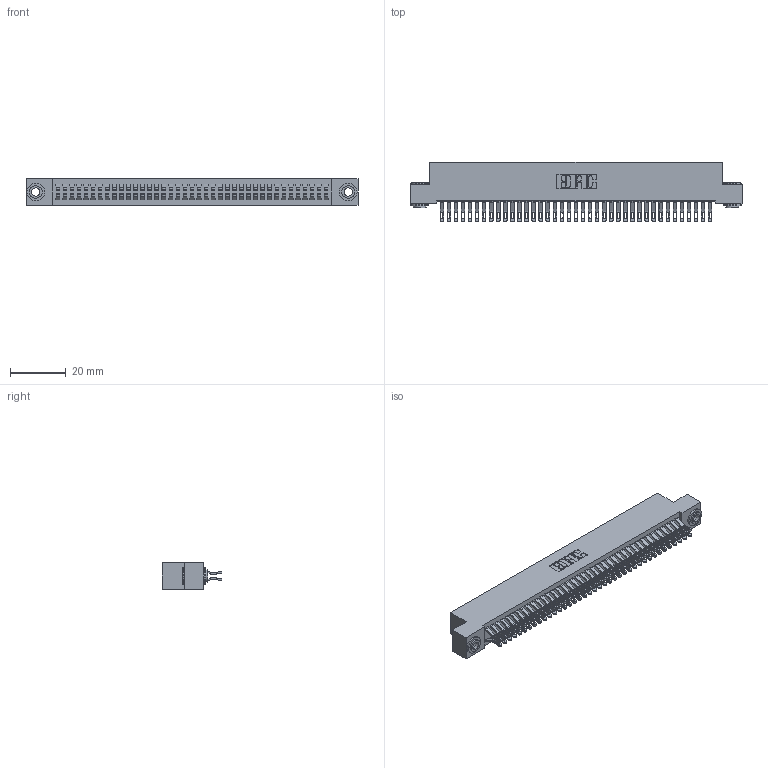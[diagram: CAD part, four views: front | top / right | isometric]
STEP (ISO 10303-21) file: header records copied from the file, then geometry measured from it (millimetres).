
FILE_DESCRIPTION (( 'STEP AP203' ), '1' );
FILE_NAME ('392-078-555-203.STEP', '2019-10-09T14:08:14', ( '' ), ( '' ), 'SwSTEP 2.0', 'SolidWorks 2016', '' );
FILE_SCHEMA (( 'CONFIG_CONTROL_DESIGN' ));
Length unit declared in the file: inch
Products named in the file (4): 342-250-002_345-250-002-102; 392-078-555-203; 342 Part_.156 TH; 345-292-001_555 Tail
Assembly tree (81 placements, depth 2):
  392-078-555-203
    342 Part_.156 TH
    345-292-001_555 Tail  x78
    342-250-002_345-250-002-102  x2
Bounding box: 119.38 x 21.47 x 9.4 mm (x, y, z)
Volume: 10951.7 mm3; surface area: 18721.4 mm2
Topology: 81 solids, 81 shells, 4672 faces, 14649 edges, 9762 vertices
Faces by surface type: plane 2728, cylinder 1936, cone 8
Entity records: 26322 total; most frequent: CARTESIAN_POINT 4375, ORIENTED_EDGE 4274, DIRECTION 3747, EDGE_CURVE 2137, LINE 1965, VECTOR 1965, VERTEX_POINT 1422, AXIS2_PLACEMENT_3D 891
